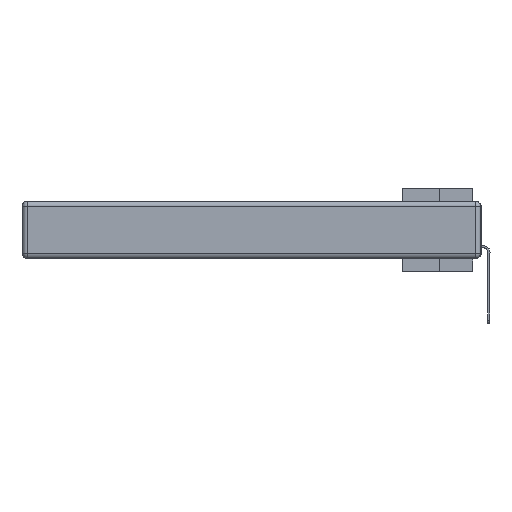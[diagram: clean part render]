
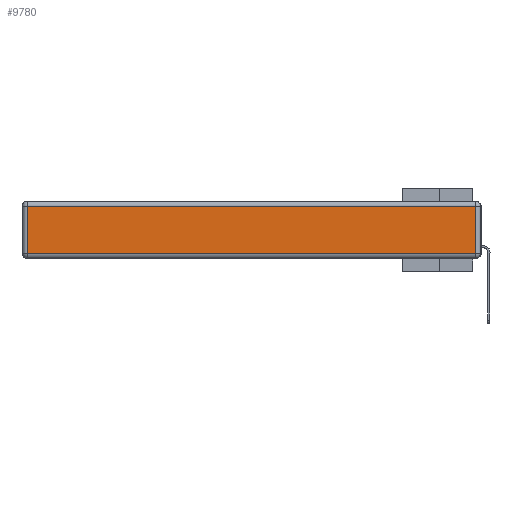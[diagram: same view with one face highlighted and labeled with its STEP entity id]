
A CAD part, left-side view. The second image highlights one B-rep face of the part: STEP entity #9780.
In plain terms, the highlighted planar face has unit normal (-1, 0, 0).
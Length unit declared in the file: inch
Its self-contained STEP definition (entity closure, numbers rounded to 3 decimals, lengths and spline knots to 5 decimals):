
#4305 = ORIENTED_EDGE ( 'NONE', *, *, #18595, .T. ) ;
#4605 = CARTESIAN_POINT ( 'NONE',  ( 0., 2.75, -0.03 ) ) ;
#4690 = EDGE_CURVE ( 'NONE', #35121, #22970, #26229, .T. ) ;
#5660 = CARTESIAN_POINT ( 'NONE',  ( 0., 0.03, -0.313 ) ) ;
#6829 = CARTESIAN_POINT ( 'NONE',  ( 0., 0.03, -0.343 ) ) ;
#7745 = VERTEX_POINT ( 'NONE', #32200 ) ;
#8027 = LINE ( 'NONE', #4605, #32296 ) ;
#8378 = CARTESIAN_POINT ( 'NONE',  ( 0., 0., -0.343 ) ) ;
#8561 = ORIENTED_EDGE ( 'NONE', *, *, #4690, .T. ) ;
#9246 = VECTOR ( 'NONE', #20053, 39.37008 ) ;
#9780 = ADVANCED_FACE ( 'NONE', ( #17446 ), #19251, .T. ) ;
#13313 = EDGE_CURVE ( 'NONE', #22970, #30391, #29071, .T. ) ;
#14211 = VECTOR ( 'NONE', #28812, 39.37008 ) ;
#15866 = ORIENTED_EDGE ( 'NONE', *, *, #23246, .T. ) ;
#16374 = CARTESIAN_POINT ( 'NONE',  ( 0., 2.72, -0.313 ) ) ;
#17335 = ORIENTED_EDGE ( 'NONE', *, *, #13313, .T. ) ;
#17446 = FACE_OUTER_BOUND ( 'NONE', #17808, .T. ) ;
#17771 = LINE ( 'NONE', #6829, #9246 ) ;
#17808 = EDGE_LOOP ( 'NONE', ( #17335, #15866, #4305, #8561 ) ) ;
#18165 = DIRECTION ( 'NONE',  ( 0., 1., 0. ) ) ;
#18595 = EDGE_CURVE ( 'NONE', #7745, #35121, #8027, .T. ) ;
#19251 = PLANE ( 'NONE',  #30415 ) ;
#20053 = DIRECTION ( 'NONE',  ( 0., 0., 1. ) ) ;
#22219 = DIRECTION ( 'NONE',  ( -1., 0., 0. ) ) ;
#22970 = VERTEX_POINT ( 'NONE', #16374 ) ;
#23246 = EDGE_CURVE ( 'NONE', #30391, #7745, #17771, .T. ) ;
#23638 = CARTESIAN_POINT ( 'NONE',  ( 0., 0., -0.313 ) ) ;
#26229 = LINE ( 'NONE', #34672, #34280 ) ;
#27659 = DIRECTION ( 'NONE',  ( 0., 0., 1. ) ) ;
#28812 = DIRECTION ( 'NONE',  ( 0., -1., 0. ) ) ;
#29071 = LINE ( 'NONE', #23638, #14211 ) ;
#29312 = DIRECTION ( 'NONE',  ( 0., 0., -1. ) ) ;
#29635 = CARTESIAN_POINT ( 'NONE',  ( 0., 2.72, -0.03 ) ) ;
#30391 = VERTEX_POINT ( 'NONE', #5660 ) ;
#30415 = AXIS2_PLACEMENT_3D ( 'NONE', #8378, #22219, #27659 ) ;
#32200 = CARTESIAN_POINT ( 'NONE',  ( 0., 0.03, -0.03 ) ) ;
#32296 = VECTOR ( 'NONE', #18165, 39.37008 ) ;
#34280 = VECTOR ( 'NONE', #29312, 39.37008 ) ;
#34672 = CARTESIAN_POINT ( 'NONE',  ( 0., 2.72, -0.343 ) ) ;
#35121 = VERTEX_POINT ( 'NONE', #29635 ) ;
